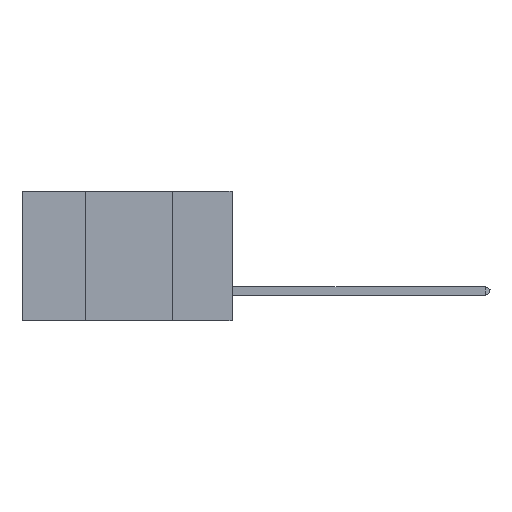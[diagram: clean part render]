
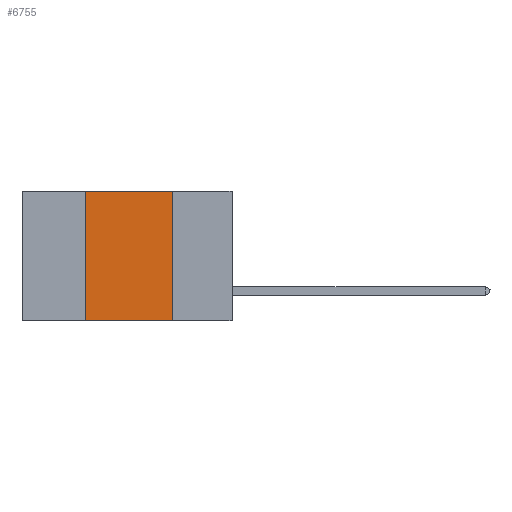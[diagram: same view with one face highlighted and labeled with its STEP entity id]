
A CAD part, left-side view. The second image highlights one B-rep face of the part: STEP entity #6755.
In plain terms, the highlighted planar face has unit normal (-1, 0, 0).
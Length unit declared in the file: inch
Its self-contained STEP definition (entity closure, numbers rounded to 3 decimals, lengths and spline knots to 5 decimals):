
#483 = DIRECTION ( 'NONE',  ( 0., 0., 1. ) ) ;
#541 = VERTEX_POINT ( 'NONE', #4625 ) ;
#656 = VECTOR ( 'NONE', #5156, 39.37008 ) ;
#778 = EDGE_CURVE ( 'NONE', #4995, #5629, #11098, .T. ) ;
#1070 = LINE ( 'NONE', #8590, #6098 ) ;
#1613 = EDGE_CURVE ( 'NONE', #5629, #541, #1070, .T. ) ;
#1638 = FACE_OUTER_BOUND ( 'NONE', #11805, .T. ) ;
#2022 = LINE ( 'NONE', #4305, #10662 ) ;
#2272 = VECTOR ( 'NONE', #483, 39.37008 ) ;
#2903 = AXIS2_PLACEMENT_3D ( 'NONE', #5352, #3116, #8844 ) ;
#3116 = DIRECTION ( 'NONE',  ( 1., 0., 0. ) ) ;
#4305 = CARTESIAN_POINT ( 'NONE',  ( 0., 0.17, 0. ) ) ;
#4405 = ORIENTED_EDGE ( 'NONE', *, *, #778, .F. ) ;
#4625 = CARTESIAN_POINT ( 'NONE',  ( 0., 0.17, 0. ) ) ;
#4995 = VERTEX_POINT ( 'NONE', #10440 ) ;
#5156 = DIRECTION ( 'NONE',  ( 0., -1., 0. ) ) ;
#5352 = CARTESIAN_POINT ( 'NONE',  ( 0., 0.6, 0. ) ) ;
#5629 = VERTEX_POINT ( 'NONE', #10792 ) ;
#5720 = ORIENTED_EDGE ( 'NONE', *, *, #1613, .F. ) ;
#5766 = EDGE_CURVE ( 'NONE', #541, #8601, #2022, .T. ) ;
#6098 = VECTOR ( 'NONE', #12132, 39.37008 ) ;
#6755 = ADVANCED_FACE ( 'NONE', ( #1638 ), #11107, .F. ) ;
#7866 = ORIENTED_EDGE ( 'NONE', *, *, #11989, .T. ) ;
#8364 = CARTESIAN_POINT ( 'NONE',  ( 0., 0.17, -0.37 ) ) ;
#8590 = CARTESIAN_POINT ( 'NONE',  ( 0., 0.6, 0. ) ) ;
#8601 = VERTEX_POINT ( 'NONE', #8364 ) ;
#8844 = DIRECTION ( 'NONE',  ( 0., 0., -1. ) ) ;
#10440 = CARTESIAN_POINT ( 'NONE',  ( 0., 0.42, -0.37 ) ) ;
#10662 = VECTOR ( 'NONE', #13553, 39.37008 ) ;
#10700 = LINE ( 'NONE', #12176, #656 ) ;
#10792 = CARTESIAN_POINT ( 'NONE',  ( 0., 0.42, 0. ) ) ;
#11098 = LINE ( 'NONE', #14268, #2272 ) ;
#11107 = PLANE ( 'NONE',  #2903 ) ;
#11130 = ORIENTED_EDGE ( 'NONE', *, *, #5766, .F. ) ;
#11805 = EDGE_LOOP ( 'NONE', ( #11130, #5720, #4405, #7866 ) ) ;
#11989 = EDGE_CURVE ( 'NONE', #4995, #8601, #10700, .T. ) ;
#12132 = DIRECTION ( 'NONE',  ( 0., -1., 0. ) ) ;
#12176 = CARTESIAN_POINT ( 'NONE',  ( 0., 0.6, -0.37 ) ) ;
#13553 = DIRECTION ( 'NONE',  ( 0., 0., -1. ) ) ;
#14268 = CARTESIAN_POINT ( 'NONE',  ( 0., 0.42, 0. ) ) ;
